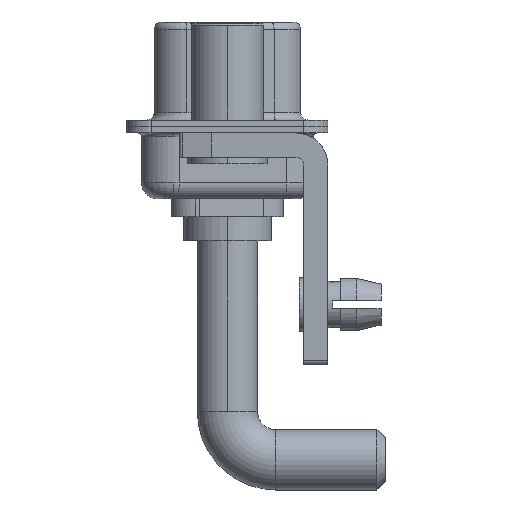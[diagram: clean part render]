
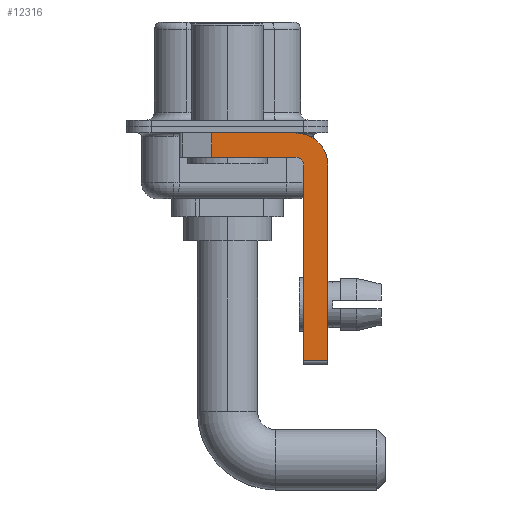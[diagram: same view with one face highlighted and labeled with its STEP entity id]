
A CAD part, left-side view. The second image highlights one B-rep face of the part: STEP entity #12316.
In plain terms, the highlighted planar face has unit normal (-1, 0, 0).
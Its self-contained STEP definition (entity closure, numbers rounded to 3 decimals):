
#192 = VECTOR ( 'NONE', #16581, 1000. ) ;
#234 = CARTESIAN_POINT ( 'NONE',  ( -2.9, -4.25, -14.55 ) ) ;
#241 = DIRECTION ( 'NONE',  ( 0., 0., -1. ) ) ;
#616 = VERTEX_POINT ( 'NONE', #3197 ) ;
#916 = EDGE_CURVE ( 'NONE', #616, #8615, #1233, .T. ) ;
#955 = EDGE_CURVE ( 'NONE', #16841, #17483, #7075, .T. ) ;
#1233 = LINE ( 'NONE', #19552, #192 ) ;
#1444 = VERTEX_POINT ( 'NONE', #13374 ) ;
#1463 = CARTESIAN_POINT ( 'NONE',  ( -2.9, -4.25, -2.4 ) ) ;
#1738 = DIRECTION ( 'NONE',  ( 0., 1., 0. ) ) ;
#2019 = LINE ( 'NONE', #4674, #4280 ) ;
#2657 = EDGE_CURVE ( 'NONE', #8615, #1444, #16167, .T. ) ;
#2764 = AXIS2_PLACEMENT_3D ( 'NONE', #8409, #17517, #4923 ) ;
#3197 = CARTESIAN_POINT ( 'NONE',  ( -2.9, -4.75, -14.55 ) ) ;
#3769 = LINE ( 'NONE', #8574, #8776 ) ;
#4280 = VECTOR ( 'NONE', #8058, 1000. ) ;
#4674 = CARTESIAN_POINT ( 'NONE',  ( -2.9, 0.978, -1.9 ) ) ;
#4923 = DIRECTION ( 'NONE',  ( 0., 0., -1. ) ) ;
#5448 = ORIENTED_EDGE ( 'NONE', *, *, #955, .F. ) ;
#5855 = CARTESIAN_POINT ( 'NONE',  ( -2.9, -6.25, -14.55 ) ) ;
#6107 = EDGE_CURVE ( 'NONE', #616, #17483, #17414, .T. ) ;
#6552 = VECTOR ( 'NONE', #15973, 1000. ) ;
#6702 = EDGE_LOOP ( 'NONE', ( #10065, #16063, #19792, #16495, #14478, #17064, #5448, #13597 ) ) ;
#6769 = PLANE ( 'NONE',  #2764 ) ;
#7075 = LINE ( 'NONE', #13308, #14237 ) ;
#7168 = DIRECTION ( 'NONE',  ( 0., 0., -1. ) ) ;
#7312 = CIRCLE ( 'NONE', #16474, 2. ) ;
#7342 = AXIS2_PLACEMENT_3D ( 'NONE', #17890, #10193, #12960 ) ;
#7429 = CARTESIAN_POINT ( 'NONE',  ( -2.9, 0.978, -1.9 ) ) ;
#7894 = FACE_OUTER_BOUND ( 'NONE', #6702, .T. ) ;
#7915 = EDGE_CURVE ( 'NONE', #1444, #9787, #12770, .T. ) ;
#8058 = DIRECTION ( 'NONE',  ( 0., 0., -1. ) ) ;
#8383 = EDGE_CURVE ( 'NONE', #11027, #9787, #2019, .T. ) ;
#8409 = CARTESIAN_POINT ( 'NONE',  ( -2.9, -4.25, -2.4 ) ) ;
#8461 = CARTESIAN_POINT ( 'NONE',  ( -2.9, -4.25, -0.4 ) ) ;
#8574 = CARTESIAN_POINT ( 'NONE',  ( -2.9, 3., -0.4 ) ) ;
#8615 = VERTEX_POINT ( 'NONE', #9886 ) ;
#8640 = VERTEX_POINT ( 'NONE', #8461 ) ;
#8776 = VECTOR ( 'NONE', #19318, 1000. ) ;
#9610 = CARTESIAN_POINT ( 'NONE',  ( -2.9, -4.25, -1.9 ) ) ;
#9703 = EDGE_CURVE ( 'NONE', #11027, #8640, #3769, .T. ) ;
#9787 = VERTEX_POINT ( 'NONE', #7429 ) ;
#9886 = CARTESIAN_POINT ( 'NONE',  ( -2.9, -4.75, -2.4 ) ) ;
#10065 = ORIENTED_EDGE ( 'NONE', *, *, #9703, .F. ) ;
#10193 = DIRECTION ( 'NONE',  ( -1., 0., 0. ) ) ;
#11027 = VERTEX_POINT ( 'NONE', #15966 ) ;
#12316 = ADVANCED_FACE ( 'NONE', ( #7894 ), #6769, .F. ) ;
#12434 = VECTOR ( 'NONE', #1738, 1000. ) ;
#12770 = LINE ( 'NONE', #9610, #12434 ) ;
#12800 = DIRECTION ( 'NONE',  ( 1., 0., 0. ) ) ;
#12960 = DIRECTION ( 'NONE',  ( 0., 0., 1. ) ) ;
#13098 = EDGE_CURVE ( 'NONE', #8640, #16841, #7312, .T. ) ;
#13308 = CARTESIAN_POINT ( 'NONE',  ( -2.9, -6.25, -2.4 ) ) ;
#13374 = CARTESIAN_POINT ( 'NONE',  ( -2.9, -4.25, -1.9 ) ) ;
#13597 = ORIENTED_EDGE ( 'NONE', *, *, #13098, .F. ) ;
#13862 = CARTESIAN_POINT ( 'NONE',  ( -2.9, -6.25, -2.4 ) ) ;
#14237 = VECTOR ( 'NONE', #7168, 1000. ) ;
#14478 = ORIENTED_EDGE ( 'NONE', *, *, #916, .F. ) ;
#15966 = CARTESIAN_POINT ( 'NONE',  ( -2.9, 0.978, -0.4 ) ) ;
#15973 = DIRECTION ( 'NONE',  ( 0., -1., 0. ) ) ;
#16063 = ORIENTED_EDGE ( 'NONE', *, *, #8383, .T. ) ;
#16167 = CIRCLE ( 'NONE', #7342, 0.5 ) ;
#16474 = AXIS2_PLACEMENT_3D ( 'NONE', #1463, #12800, #241 ) ;
#16495 = ORIENTED_EDGE ( 'NONE', *, *, #2657, .F. ) ;
#16581 = DIRECTION ( 'NONE',  ( 0., 0., 1. ) ) ;
#16841 = VERTEX_POINT ( 'NONE', #13862 ) ;
#17064 = ORIENTED_EDGE ( 'NONE', *, *, #6107, .T. ) ;
#17414 = LINE ( 'NONE', #234, #6552 ) ;
#17483 = VERTEX_POINT ( 'NONE', #5855 ) ;
#17517 = DIRECTION ( 'NONE',  ( 1., 0., 0. ) ) ;
#17890 = CARTESIAN_POINT ( 'NONE',  ( -2.9, -4.25, -2.4 ) ) ;
#19318 = DIRECTION ( 'NONE',  ( 0., -1., 0. ) ) ;
#19552 = CARTESIAN_POINT ( 'NONE',  ( -2.9, -4.75, -14.8 ) ) ;
#19792 = ORIENTED_EDGE ( 'NONE', *, *, #7915, .F. ) ;
